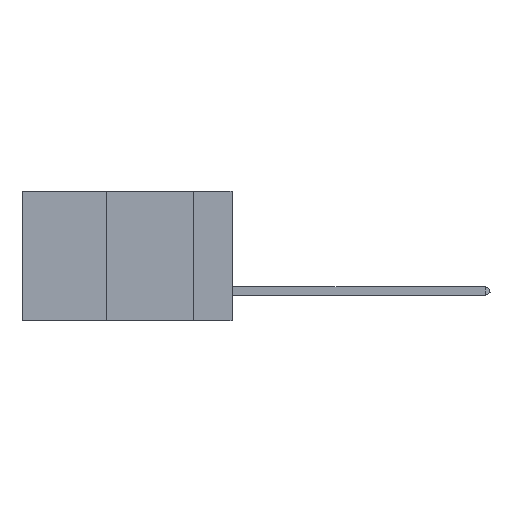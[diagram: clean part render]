
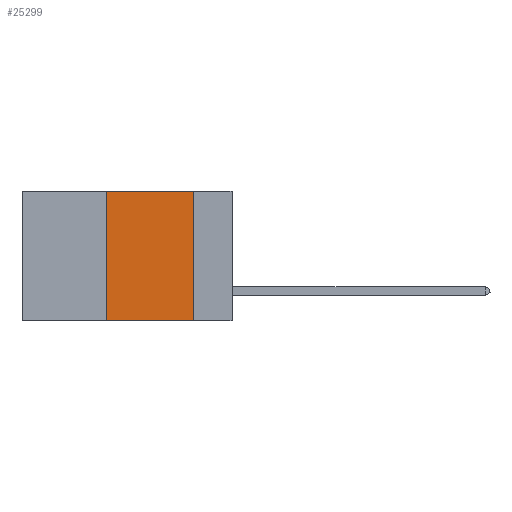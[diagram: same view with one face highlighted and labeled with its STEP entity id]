
A CAD part, left-side view. The second image highlights one B-rep face of the part: STEP entity #25299.
In plain terms, the highlighted planar face has unit normal (-1, 0, 0).
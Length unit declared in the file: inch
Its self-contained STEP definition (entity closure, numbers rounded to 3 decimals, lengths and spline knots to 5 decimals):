
#5371 = CARTESIAN_POINT ( 'NONE',  ( 0., 0.36, -0.37 ) ) ;
#8382 = EDGE_CURVE ( 'NONE', #42072, #15686, #18629, .T. ) ;
#8731 = LINE ( 'NONE', #22682, #47913 ) ;
#12156 = DIRECTION ( 'NONE',  ( 0., 0., -1. ) ) ;
#14926 = AXIS2_PLACEMENT_3D ( 'NONE', #35442, #47255, #12156 ) ;
#15657 = EDGE_CURVE ( 'NONE', #47238, #42072, #25272, .T. ) ;
#15686 = VERTEX_POINT ( 'NONE', #33673 ) ;
#16652 = ORIENTED_EDGE ( 'NONE', *, *, #8382, .F. ) ;
#16925 = EDGE_CURVE ( 'NONE', #49298, #47238, #8731, .T. ) ;
#18629 = LINE ( 'NONE', #47386, #29666 ) ;
#22161 = CARTESIAN_POINT ( 'NONE',  ( 0., 0.11, 0. ) ) ;
#22350 = DIRECTION ( 'NONE',  ( 0., -1., 0. ) ) ;
#22682 = CARTESIAN_POINT ( 'NONE',  ( 0., 0.36, 0. ) ) ;
#25272 = LINE ( 'NONE', #38123, #33898 ) ;
#25299 = ADVANCED_FACE ( 'NONE', ( #32719 ), #28078, .F. ) ;
#28078 = PLANE ( 'NONE',  #14926 ) ;
#29666 = VECTOR ( 'NONE', #31630, 39.37008 ) ;
#30335 = CARTESIAN_POINT ( 'NONE',  ( 0., 0.36, 0. ) ) ;
#31630 = DIRECTION ( 'NONE',  ( 0., 0., -1. ) ) ;
#32719 = FACE_OUTER_BOUND ( 'NONE', #37923, .T. ) ;
#33673 = CARTESIAN_POINT ( 'NONE',  ( 0., 0.11, -0.37 ) ) ;
#33898 = VECTOR ( 'NONE', #22350, 39.37008 ) ;
#35442 = CARTESIAN_POINT ( 'NONE',  ( 0., 0.6, 0. ) ) ;
#36534 = DIRECTION ( 'NONE',  ( 0., -1., 0. ) ) ;
#37923 = EDGE_LOOP ( 'NONE', ( #16652, #48960, #46789, #38188 ) ) ;
#37942 = DIRECTION ( 'NONE',  ( 0., 0., 1. ) ) ;
#38123 = CARTESIAN_POINT ( 'NONE',  ( 0., 0.6, 0. ) ) ;
#38188 = ORIENTED_EDGE ( 'NONE', *, *, #40434, .T. ) ;
#38262 = VECTOR ( 'NONE', #36534, 39.37008 ) ;
#40434 = EDGE_CURVE ( 'NONE', #49298, #15686, #41343, .T. ) ;
#40512 = CARTESIAN_POINT ( 'NONE',  ( 0., 0.6, -0.37 ) ) ;
#41343 = LINE ( 'NONE', #40512, #38262 ) ;
#42072 = VERTEX_POINT ( 'NONE', #22161 ) ;
#46789 = ORIENTED_EDGE ( 'NONE', *, *, #16925, .F. ) ;
#47238 = VERTEX_POINT ( 'NONE', #30335 ) ;
#47255 = DIRECTION ( 'NONE',  ( 1., 0., 0. ) ) ;
#47386 = CARTESIAN_POINT ( 'NONE',  ( 0., 0.11, 0. ) ) ;
#47913 = VECTOR ( 'NONE', #37942, 39.37008 ) ;
#48960 = ORIENTED_EDGE ( 'NONE', *, *, #15657, .F. ) ;
#49298 = VERTEX_POINT ( 'NONE', #5371 ) ;
